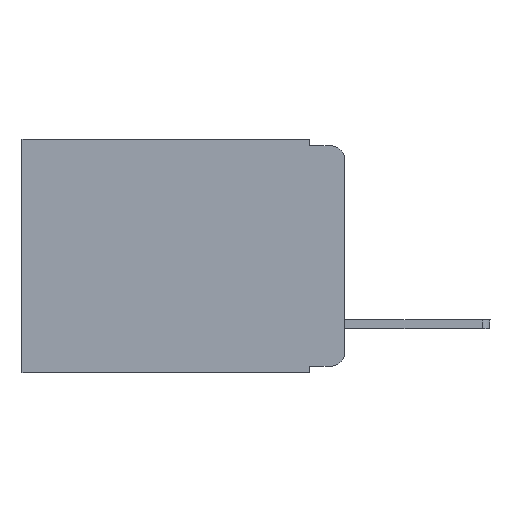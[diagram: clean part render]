
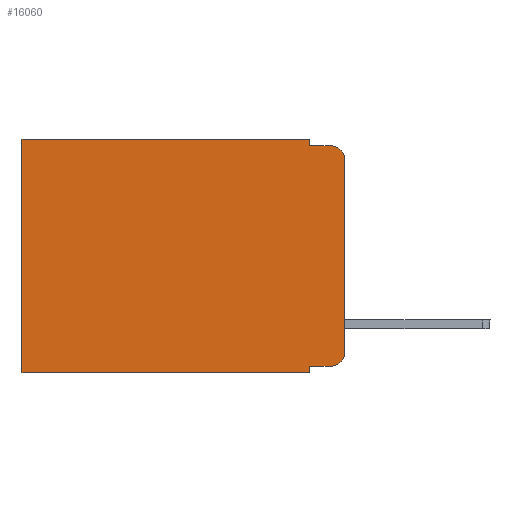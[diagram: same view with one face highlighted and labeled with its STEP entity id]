
A CAD part, left-side view. The second image highlights one B-rep face of the part: STEP entity #16060.
In plain terms, the highlighted planar face has unit normal (-1, 0, 0).
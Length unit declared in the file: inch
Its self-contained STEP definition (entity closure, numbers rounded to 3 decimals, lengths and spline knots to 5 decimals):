
#455 = PLANE ( 'NONE',  #22318 ) ;
#520 = VECTOR ( 'NONE', #8823, 39.37008 ) ;
#540 = DIRECTION ( 'NONE',  ( 0., 0., -1. ) ) ;
#969 = EDGE_CURVE ( 'NONE', #9413, #22063, #7953, .T. ) ;
#1209 = LINE ( 'NONE', #23173, #10997 ) ;
#1254 = LINE ( 'NONE', #20450, #4418 ) ;
#1860 = DIRECTION ( 'NONE',  ( 0., -1., 0. ) ) ;
#1956 = CIRCLE ( 'NONE', #10047, 0.02 ) ;
#2037 = ORIENTED_EDGE ( 'NONE', *, *, #14852, .F. ) ;
#3088 = EDGE_LOOP ( 'NONE', ( #2037, #6000, #14285, #5051, #14806, #15401, #20506, #3982, #4619, #22141 ) ) ;
#3125 = CARTESIAN_POINT ( 'NONE',  ( 0.298, 0.051, -0.333 ) ) ;
#3168 = EDGE_CURVE ( 'NONE', #18233, #5169, #13118, .T. ) ;
#3982 = ORIENTED_EDGE ( 'NONE', *, *, #13201, .F. ) ;
#4342 = CARTESIAN_POINT ( 'NONE',  ( 0.298, 0.051, -0.01 ) ) ;
#4418 = VECTOR ( 'NONE', #1860, 39.37008 ) ;
#4430 = EDGE_CURVE ( 'NONE', #6849, #13403, #1254, .T. ) ;
#4562 = VECTOR ( 'NONE', #19671, 39.37008 ) ;
#4563 = LINE ( 'NONE', #7877, #18133 ) ;
#4591 = FACE_OUTER_BOUND ( 'NONE', #3088, .T. ) ;
#4619 = ORIENTED_EDGE ( 'NONE', *, *, #4430, .T. ) ;
#4655 = CARTESIAN_POINT ( 'NONE',  ( 0.298, 0., 0. ) ) ;
#5051 = ORIENTED_EDGE ( 'NONE', *, *, #3168, .F. ) ;
#5169 = VERTEX_POINT ( 'NONE', #4342 ) ;
#5438 = CARTESIAN_POINT ( 'NONE',  ( 0.298, 0.02, -0.01 ) ) ;
#5444 = EDGE_CURVE ( 'NONE', #5169, #21723, #1209, .T. ) ;
#5545 = VERTEX_POINT ( 'NONE', #10373 ) ;
#6000 = ORIENTED_EDGE ( 'NONE', *, *, #14757, .T. ) ;
#6043 = DIRECTION ( 'NONE',  ( 1., 0., 0. ) ) ;
#6271 = DIRECTION ( 'NONE',  ( 0., 0., -1. ) ) ;
#6843 = DIRECTION ( 'NONE',  ( 0., -1., 0. ) ) ;
#6849 = VERTEX_POINT ( 'NONE', #3125 ) ;
#7288 = EDGE_CURVE ( 'NONE', #18233, #9413, #19880, .T. ) ;
#7456 = EDGE_CURVE ( 'NONE', #17658, #22063, #11486, .T. ) ;
#7877 = CARTESIAN_POINT ( 'NONE',  ( 0.298, 0., 0. ) ) ;
#7953 = LINE ( 'NONE', #8347, #14352 ) ;
#8347 = CARTESIAN_POINT ( 'NONE',  ( 0.298, 0.473, 0. ) ) ;
#8823 = DIRECTION ( 'NONE',  ( 0., 1., 0. ) ) ;
#9024 = CARTESIAN_POINT ( 'NONE',  ( 0.298, 0.051, 0. ) ) ;
#9413 = VERTEX_POINT ( 'NONE', #12081 ) ;
#9980 = CARTESIAN_POINT ( 'NONE',  ( 0.298, 0.051, -0.343 ) ) ;
#10047 = AXIS2_PLACEMENT_3D ( 'NONE', #20828, #20501, #17012 ) ;
#10373 = CARTESIAN_POINT ( 'NONE',  ( 0.298, 0., -0.313 ) ) ;
#10384 = LINE ( 'NONE', #11882, #20251 ) ;
#10490 = CARTESIAN_POINT ( 'NONE',  ( 0.298, 0., -0.03 ) ) ;
#10997 = VECTOR ( 'NONE', #6843, 39.37008 ) ;
#11031 = DIRECTION ( 'NONE',  ( 0., 0., -1. ) ) ;
#11112 = VECTOR ( 'NONE', #11031, 39.37008 ) ;
#11453 = VERTEX_POINT ( 'NONE', #10490 ) ;
#11486 = LINE ( 'NONE', #19913, #520 ) ;
#11882 = CARTESIAN_POINT ( 'NONE',  ( 0.298, 0.051, 0. ) ) ;
#12081 = CARTESIAN_POINT ( 'NONE',  ( 0.298, 0.473, 0. ) ) ;
#13118 = LINE ( 'NONE', #9024, #11112 ) ;
#13201 = EDGE_CURVE ( 'NONE', #6849, #17658, #10384, .T. ) ;
#13379 = CARTESIAN_POINT ( 'NONE',  ( 0.298, 0., 0. ) ) ;
#13403 = VERTEX_POINT ( 'NONE', #17235 ) ;
#14285 = ORIENTED_EDGE ( 'NONE', *, *, #5444, .F. ) ;
#14352 = VECTOR ( 'NONE', #15651, 39.37008 ) ;
#14757 = EDGE_CURVE ( 'NONE', #11453, #21723, #1956, .T. ) ;
#14793 = CIRCLE ( 'NONE', #19101, 0.02 ) ;
#14806 = ORIENTED_EDGE ( 'NONE', *, *, #7288, .T. ) ;
#14852 = EDGE_CURVE ( 'NONE', #11453, #5545, #4563, .T. ) ;
#15323 = CARTESIAN_POINT ( 'NONE',  ( 0.298, 0.02, -0.313 ) ) ;
#15401 = ORIENTED_EDGE ( 'NONE', *, *, #969, .T. ) ;
#15651 = DIRECTION ( 'NONE',  ( 0., 0., -1. ) ) ;
#16060 = ADVANCED_FACE ( 'NONE', ( #4591 ), #455, .F. ) ;
#17012 = DIRECTION ( 'NONE',  ( 0., 0., -1. ) ) ;
#17235 = CARTESIAN_POINT ( 'NONE',  ( 0.298, 0.02, -0.333 ) ) ;
#17366 = CARTESIAN_POINT ( 'NONE',  ( 0.298, 0.473, -0.343 ) ) ;
#17590 = CARTESIAN_POINT ( 'NONE',  ( 0.298, 0.051, 0. ) ) ;
#17658 = VERTEX_POINT ( 'NONE', #9980 ) ;
#18133 = VECTOR ( 'NONE', #22359, 39.37008 ) ;
#18233 = VERTEX_POINT ( 'NONE', #17590 ) ;
#19064 = DIRECTION ( 'NONE',  ( -1., 0., 0. ) ) ;
#19101 = AXIS2_PLACEMENT_3D ( 'NONE', #15323, #19064, #6271 ) ;
#19671 = DIRECTION ( 'NONE',  ( 0., 1., 0. ) ) ;
#19880 = LINE ( 'NONE', #4655, #4562 ) ;
#19913 = CARTESIAN_POINT ( 'NONE',  ( 0.298, 0., -0.343 ) ) ;
#20227 = EDGE_CURVE ( 'NONE', #13403, #5545, #14793, .T. ) ;
#20251 = VECTOR ( 'NONE', #22732, 39.37008 ) ;
#20450 = CARTESIAN_POINT ( 'NONE',  ( 0.298, 0.051, -0.333 ) ) ;
#20501 = DIRECTION ( 'NONE',  ( -1., 0., 0. ) ) ;
#20506 = ORIENTED_EDGE ( 'NONE', *, *, #7456, .F. ) ;
#20828 = CARTESIAN_POINT ( 'NONE',  ( 0.298, 0.02, -0.03 ) ) ;
#21723 = VERTEX_POINT ( 'NONE', #5438 ) ;
#22063 = VERTEX_POINT ( 'NONE', #17366 ) ;
#22141 = ORIENTED_EDGE ( 'NONE', *, *, #20227, .T. ) ;
#22318 = AXIS2_PLACEMENT_3D ( 'NONE', #13379, #6043, #540 ) ;
#22359 = DIRECTION ( 'NONE',  ( 0., 0., -1. ) ) ;
#22732 = DIRECTION ( 'NONE',  ( 0., 0., -1. ) ) ;
#23173 = CARTESIAN_POINT ( 'NONE',  ( 0.298, 0.051, -0.01 ) ) ;
